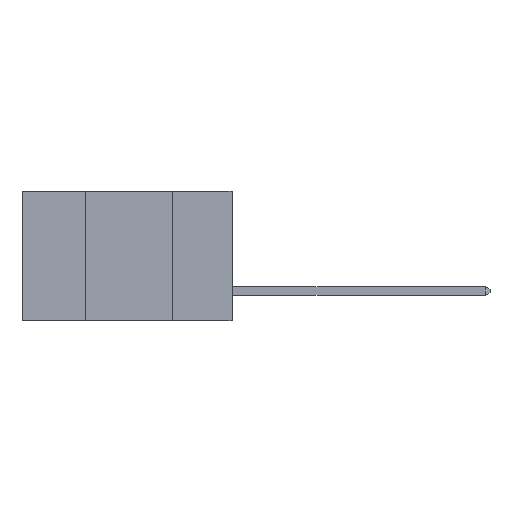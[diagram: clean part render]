
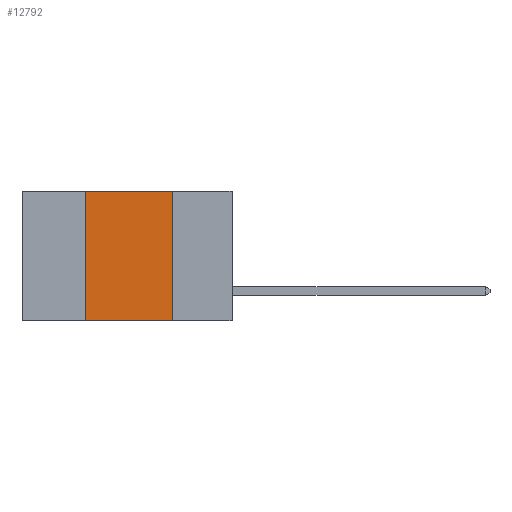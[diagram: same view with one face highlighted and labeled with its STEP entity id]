
A CAD part, left-side view. The second image highlights one B-rep face of the part: STEP entity #12792.
In plain terms, the highlighted planar face has unit normal (-1, 0, 0).
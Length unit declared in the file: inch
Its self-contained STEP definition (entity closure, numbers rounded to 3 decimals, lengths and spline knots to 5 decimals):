
#898 = ORIENTED_EDGE ( 'NONE', *, *, #15856, .T. ) ;
#1262 = DIRECTION ( 'NONE',  ( 0., 0., -1. ) ) ;
#2822 = ORIENTED_EDGE ( 'NONE', *, *, #15946, .F. ) ;
#2971 = CARTESIAN_POINT ( 'NONE',  ( 0., 0.42, 0. ) ) ;
#3221 = PLANE ( 'NONE',  #4848 ) ;
#3273 = CARTESIAN_POINT ( 'NONE',  ( 0., 0.17, -0.37 ) ) ;
#3287 = DIRECTION ( 'NONE',  ( 0., 0., -1. ) ) ;
#3529 = LINE ( 'NONE', #9132, #19323 ) ;
#4845 = VERTEX_POINT ( 'NONE', #16511 ) ;
#4848 = AXIS2_PLACEMENT_3D ( 'NONE', #9350, #12277, #3287 ) ;
#4992 = VERTEX_POINT ( 'NONE', #12862 ) ;
#6173 = CARTESIAN_POINT ( 'NONE',  ( 0., 0.6, -0.37 ) ) ;
#7073 = LINE ( 'NONE', #8837, #14480 ) ;
#8135 = VERTEX_POINT ( 'NONE', #3273 ) ;
#8545 = VECTOR ( 'NONE', #13839, 39.37008 ) ;
#8837 = CARTESIAN_POINT ( 'NONE',  ( 0., 0.17, 0. ) ) ;
#9132 = CARTESIAN_POINT ( 'NONE',  ( 0., 0.42, 0. ) ) ;
#9350 = CARTESIAN_POINT ( 'NONE',  ( 0., 0.6, 0. ) ) ;
#10683 = DIRECTION ( 'NONE',  ( 0., -1., 0. ) ) ;
#11546 = EDGE_CURVE ( 'NONE', #4845, #13973, #3529, .T. ) ;
#11918 = FACE_OUTER_BOUND ( 'NONE', #13643, .T. ) ;
#12277 = DIRECTION ( 'NONE',  ( 1., 0., 0. ) ) ;
#12346 = CARTESIAN_POINT ( 'NONE',  ( 0., 0.6, 0. ) ) ;
#12474 = LINE ( 'NONE', #12346, #8545 ) ;
#12792 = ADVANCED_FACE ( 'NONE', ( #11918 ), #3221, .F. ) ;
#12862 = CARTESIAN_POINT ( 'NONE',  ( 0., 0.17, 0. ) ) ;
#13643 = EDGE_LOOP ( 'NONE', ( #17500, #2822, #15929, #898 ) ) ;
#13839 = DIRECTION ( 'NONE',  ( 0., -1., 0. ) ) ;
#13973 = VERTEX_POINT ( 'NONE', #2971 ) ;
#14315 = LINE ( 'NONE', #6173, #17770 ) ;
#14480 = VECTOR ( 'NONE', #1262, 39.37008 ) ;
#15856 = EDGE_CURVE ( 'NONE', #4845, #8135, #14315, .T. ) ;
#15929 = ORIENTED_EDGE ( 'NONE', *, *, #11546, .F. ) ;
#15946 = EDGE_CURVE ( 'NONE', #13973, #4992, #12474, .T. ) ;
#16511 = CARTESIAN_POINT ( 'NONE',  ( 0., 0.42, -0.37 ) ) ;
#17451 = EDGE_CURVE ( 'NONE', #4992, #8135, #7073, .T. ) ;
#17500 = ORIENTED_EDGE ( 'NONE', *, *, #17451, .F. ) ;
#17770 = VECTOR ( 'NONE', #10683, 39.37008 ) ;
#19323 = VECTOR ( 'NONE', #19378, 39.37008 ) ;
#19378 = DIRECTION ( 'NONE',  ( 0., 0., 1. ) ) ;
